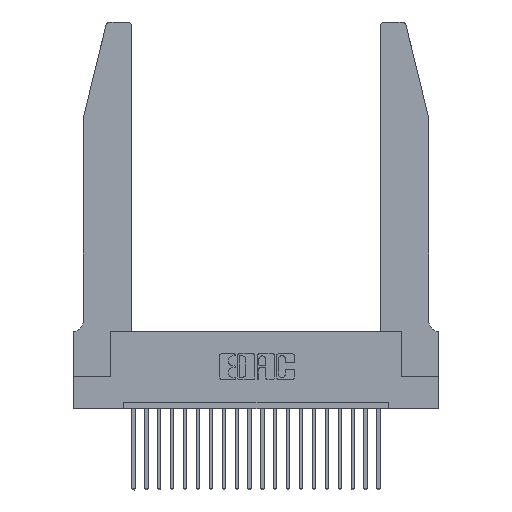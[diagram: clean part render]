
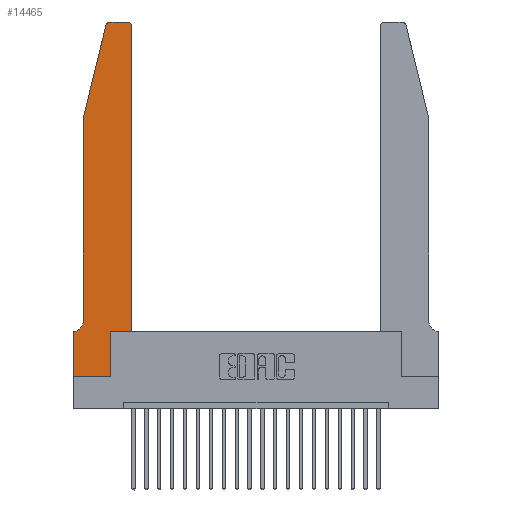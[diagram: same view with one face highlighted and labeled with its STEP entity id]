
A CAD part, top view. The second image highlights one B-rep face of the part: STEP entity #14465.
In plain terms, the highlighted planar face has unit normal (0, 0, 1).
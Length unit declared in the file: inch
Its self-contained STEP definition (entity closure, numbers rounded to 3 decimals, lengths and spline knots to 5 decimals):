
#81 = VECTOR ( 'NONE', #7093, 39.37008 ) ;
#307 = DIRECTION ( 'NONE',  ( 1., 0., 0. ) ) ;
#365 = EDGE_CURVE ( 'NONE', #14766, #15071, #6516, .T. ) ;
#804 = CARTESIAN_POINT ( 'NONE',  ( 0.2865, 0., 0.37 ) ) ;
#840 = CARTESIAN_POINT ( 'NONE',  ( 0.0755, 2., 0.37 ) ) ;
#1923 = CARTESIAN_POINT ( 'NONE',  ( 0., 0.35, 0.37 ) ) ;
#2000 = CARTESIAN_POINT ( 'NONE',  ( 0.4205, 2.72, 0.37 ) ) ;
#2720 = CARTESIAN_POINT ( 'NONE',  ( 0.0755, 0.35, 0.37 ) ) ;
#2760 = LINE ( 'NONE', #18034, #7966 ) ;
#2788 = LINE ( 'NONE', #10475, #5814 ) ;
#3408 = AXIS2_PLACEMENT_3D ( 'NONE', #14041, #17745, #7173 ) ;
#3555 = CARTESIAN_POINT ( 'NONE',  ( 0.0755, 2., 0.37 ) ) ;
#3789 = CIRCLE ( 'NONE', #6990, 0.03 ) ;
#3834 = VERTEX_POINT ( 'NONE', #14124 ) ;
#3836 = EDGE_CURVE ( 'NONE', #4990, #7536, #12187, .T. ) ;
#4257 = DIRECTION ( 'NONE',  ( 0., 0., 1. ) ) ;
#4408 = EDGE_CURVE ( 'NONE', #14760, #6121, #2788, .T. ) ;
#4459 = EDGE_CURVE ( 'NONE', #5553, #18178, #20957, .T. ) ;
#4637 = EDGE_CURVE ( 'NONE', #3834, #4990, #17136, .T. ) ;
#4728 = CARTESIAN_POINT ( 'NONE',  ( 0.0055, 0.42, 0.37 ) ) ;
#4895 = DIRECTION ( 'NONE',  ( 0., 1., 0. ) ) ;
#4990 = VERTEX_POINT ( 'NONE', #7057 ) ;
#5553 = VERTEX_POINT ( 'NONE', #1923 ) ;
#5665 = AXIS2_PLACEMENT_3D ( 'NONE', #16521, #4257, #11103 ) ;
#5739 = VERTEX_POINT ( 'NONE', #21888 ) ;
#5793 = VECTOR ( 'NONE', #19252, 39.37008 ) ;
#5814 = VECTOR ( 'NONE', #4895, 39.37008 ) ;
#5940 = DIRECTION ( 'NONE',  ( 1., 0., 0. ) ) ;
#6027 = ORIENTED_EDGE ( 'NONE', *, *, #11467, .T. ) ;
#6121 = VERTEX_POINT ( 'NONE', #18523 ) ;
#6516 = CIRCLE ( 'NONE', #16668, 0.07 ) ;
#6923 = VECTOR ( 'NONE', #20116, 39.37008 ) ;
#6990 = AXIS2_PLACEMENT_3D ( 'NONE', #2000, #14374, #12757 ) ;
#7057 = CARTESIAN_POINT ( 'NONE',  ( 0.25487, 2.72718, 0.37 ) ) ;
#7093 = DIRECTION ( 'NONE',  ( -0.239, -0.971, 0. ) ) ;
#7173 = DIRECTION ( 'NONE',  ( 1., 0., 0. ) ) ;
#7320 = DIRECTION ( 'NONE',  ( -1., 0., 0. ) ) ;
#7322 = LINE ( 'NONE', #2720, #11196 ) ;
#7483 = ORIENTED_EDGE ( 'NONE', *, *, #9088, .T. ) ;
#7536 = VERTEX_POINT ( 'NONE', #840 ) ;
#7762 = PLANE ( 'NONE',  #5665 ) ;
#7926 = CARTESIAN_POINT ( 'NONE',  ( 0.0755, 0.42, 0.37 ) ) ;
#7934 = DIRECTION ( 'NONE',  ( 0., 1., 0. ) ) ;
#7966 = VECTOR ( 'NONE', #5940, 39.37008 ) ;
#8068 = CARTESIAN_POINT ( 'NONE',  ( 0.4505, 0.35, 0.37 ) ) ;
#9088 = EDGE_CURVE ( 'NONE', #15071, #5553, #7322, .T. ) ;
#9746 = ORIENTED_EDGE ( 'NONE', *, *, #14562, .T. ) ;
#10475 = CARTESIAN_POINT ( 'NONE',  ( 0.4505, 0.35, 0.37 ) ) ;
#10713 = CARTESIAN_POINT ( 'NONE',  ( 0.0755, 2., 0.37 ) ) ;
#10799 = LINE ( 'NONE', #11244, #6923 ) ;
#10928 = FACE_OUTER_BOUND ( 'NONE', #22302, .T. ) ;
#11103 = DIRECTION ( 'NONE',  ( 1., 0., 0. ) ) ;
#11196 = VECTOR ( 'NONE', #7320, 39.37008 ) ;
#11244 = CARTESIAN_POINT ( 'NONE',  ( 0.2605, 2.75, 0.37 ) ) ;
#11467 = EDGE_CURVE ( 'NONE', #18178, #12789, #21800, .T. ) ;
#12048 = ORIENTED_EDGE ( 'NONE', *, *, #365, .T. ) ;
#12187 = LINE ( 'NONE', #10713, #81 ) ;
#12629 = CARTESIAN_POINT ( 'NONE',  ( 0., 0., 0.37 ) ) ;
#12716 = EDGE_CURVE ( 'NONE', #13509, #14760, #2760, .T. ) ;
#12757 = DIRECTION ( 'NONE',  ( 1., 0., 0. ) ) ;
#12789 = VERTEX_POINT ( 'NONE', #804 ) ;
#12904 = EDGE_CURVE ( 'NONE', #7536, #14766, #18727, .T. ) ;
#13059 = CARTESIAN_POINT ( 'NONE',  ( 0.2865, 0.35, 0.37 ) ) ;
#13509 = VERTEX_POINT ( 'NONE', #13059 ) ;
#13543 = ORIENTED_EDGE ( 'NONE', *, *, #4408, .T. ) ;
#13822 = VECTOR ( 'NONE', #307, 39.37008 ) ;
#14041 = CARTESIAN_POINT ( 'NONE',  ( 0.284, 2.72, 0.37 ) ) ;
#14120 = ORIENTED_EDGE ( 'NONE', *, *, #4637, .T. ) ;
#14124 = CARTESIAN_POINT ( 'NONE',  ( 0.284, 2.75, 0.37 ) ) ;
#14374 = DIRECTION ( 'NONE',  ( 0., 0., 1. ) ) ;
#14465 = ADVANCED_FACE ( 'NONE', ( #10928 ), #7762, .T. ) ;
#14562 = EDGE_CURVE ( 'NONE', #6121, #5739, #3789, .T. ) ;
#14760 = VERTEX_POINT ( 'NONE', #8068 ) ;
#14766 = VERTEX_POINT ( 'NONE', #7926 ) ;
#15071 = VERTEX_POINT ( 'NONE', #21726 ) ;
#15134 = ORIENTED_EDGE ( 'NONE', *, *, #3836, .T. ) ;
#15797 = VECTOR ( 'NONE', #7934, 39.37008 ) ;
#16031 = VECTOR ( 'NONE', #19916, 39.37008 ) ;
#16182 = ORIENTED_EDGE ( 'NONE', *, *, #22149, .T. ) ;
#16521 = CARTESIAN_POINT ( 'NONE',  ( 0., 0.35, 0.37 ) ) ;
#16556 = ORIENTED_EDGE ( 'NONE', *, *, #4459, .T. ) ;
#16668 = AXIS2_PLACEMENT_3D ( 'NONE', #4728, #22191, #16973 ) ;
#16750 = CARTESIAN_POINT ( 'NONE',  ( 0.2865, 0.35, 0.37 ) ) ;
#16973 = DIRECTION ( 'NONE',  ( -1., 0., 0. ) ) ;
#17136 = CIRCLE ( 'NONE', #3408, 0.03 ) ;
#17209 = ORIENTED_EDGE ( 'NONE', *, *, #21584, .T. ) ;
#17745 = DIRECTION ( 'NONE',  ( 0., 0., 1. ) ) ;
#18034 = CARTESIAN_POINT ( 'NONE',  ( 0.4505, 0.35, 0.37 ) ) ;
#18178 = VERTEX_POINT ( 'NONE', #12629 ) ;
#18523 = CARTESIAN_POINT ( 'NONE',  ( 0.4505, 2.72, 0.37 ) ) ;
#18727 = LINE ( 'NONE', #3555, #5793 ) ;
#19199 = ORIENTED_EDGE ( 'NONE', *, *, #12716, .T. ) ;
#19252 = DIRECTION ( 'NONE',  ( 0., -1., 0. ) ) ;
#19916 = DIRECTION ( 'NONE',  ( 0., -1., 0. ) ) ;
#19950 = LINE ( 'NONE', #16750, #15797 ) ;
#20116 = DIRECTION ( 'NONE',  ( -1., 0., 0. ) ) ;
#20957 = LINE ( 'NONE', #21214, #16031 ) ;
#21214 = CARTESIAN_POINT ( 'NONE',  ( 0., 0., 0.37 ) ) ;
#21378 = CARTESIAN_POINT ( 'NONE',  ( 0., 0., 0.37 ) ) ;
#21584 = EDGE_CURVE ( 'NONE', #12789, #13509, #19950, .T. ) ;
#21726 = CARTESIAN_POINT ( 'NONE',  ( 0.0055, 0.35, 0.37 ) ) ;
#21800 = LINE ( 'NONE', #21378, #13822 ) ;
#21888 = CARTESIAN_POINT ( 'NONE',  ( 0.4205, 2.75, 0.37 ) ) ;
#22000 = ORIENTED_EDGE ( 'NONE', *, *, #12904, .T. ) ;
#22149 = EDGE_CURVE ( 'NONE', #5739, #3834, #10799, .T. ) ;
#22191 = DIRECTION ( 'NONE',  ( 0., 0., -1. ) ) ;
#22302 = EDGE_LOOP ( 'NONE', ( #16182, #14120, #15134, #22000, #12048, #7483, #16556, #6027, #17209, #19199, #13543, #9746 ) ) ;
